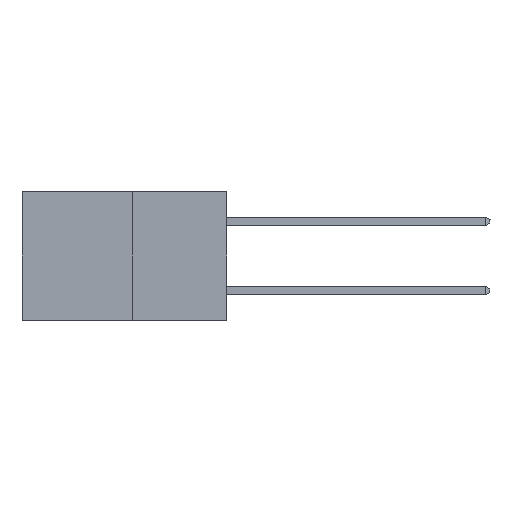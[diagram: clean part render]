
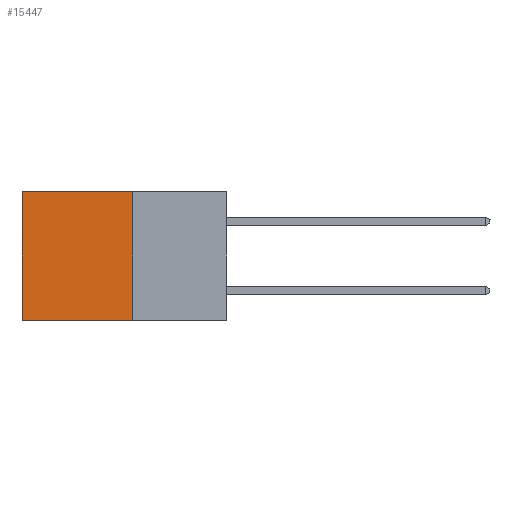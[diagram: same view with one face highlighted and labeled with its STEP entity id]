
A CAD part, left-side view. The second image highlights one B-rep face of the part: STEP entity #15447.
In plain terms, the highlighted planar face has unit normal (-1, 0, 0).
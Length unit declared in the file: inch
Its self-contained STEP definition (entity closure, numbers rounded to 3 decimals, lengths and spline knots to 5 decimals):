
#273 = FACE_OUTER_BOUND ( 'NONE', #14541, .T. ) ;
#446 = DIRECTION ( 'NONE',  ( 1., 0., 0. ) ) ;
#897 = EDGE_CURVE ( 'NONE', #8844, #6362, #9414, .T. ) ;
#1646 = CARTESIAN_POINT ( 'NONE',  ( 0.277, 0.59, -0.37 ) ) ;
#2128 = DIRECTION ( 'NONE',  ( 0., 1., 0. ) ) ;
#2238 = DIRECTION ( 'NONE',  ( 0., 0., -1. ) ) ;
#2495 = CARTESIAN_POINT ( 'NONE',  ( 0.277, 0.59, -0.37 ) ) ;
#2591 = CARTESIAN_POINT ( 'NONE',  ( 0.277, 0.27, -0.37 ) ) ;
#2794 = DIRECTION ( 'NONE',  ( 0., 1., 0. ) ) ;
#3604 = VECTOR ( 'NONE', #2794, 39.37008 ) ;
#4494 = LINE ( 'NONE', #2591, #3604 ) ;
#5032 = CARTESIAN_POINT ( 'NONE',  ( 0.277, 0.59, 0. ) ) ;
#5323 = LINE ( 'NONE', #15180, #15571 ) ;
#6038 = VECTOR ( 'NONE', #14435, 39.37008 ) ;
#6362 = VERTEX_POINT ( 'NONE', #15870 ) ;
#6744 = EDGE_CURVE ( 'NONE', #6362, #9347, #4494, .T. ) ;
#6822 = LINE ( 'NONE', #1646, #17434 ) ;
#7029 = VERTEX_POINT ( 'NONE', #5032 ) ;
#7453 = EDGE_CURVE ( 'NONE', #7029, #9347, #6822, .T. ) ;
#7504 = ORIENTED_EDGE ( 'NONE', *, *, #6744, .F. ) ;
#7928 = AXIS2_PLACEMENT_3D ( 'NONE', #13498, #446, #10574 ) ;
#8844 = VERTEX_POINT ( 'NONE', #16671 ) ;
#9106 = PLANE ( 'NONE',  #7928 ) ;
#9347 = VERTEX_POINT ( 'NONE', #2495 ) ;
#9414 = LINE ( 'NONE', #13975, #6038 ) ;
#10574 = DIRECTION ( 'NONE',  ( 0., 0., -1. ) ) ;
#12203 = ORIENTED_EDGE ( 'NONE', *, *, #12925, .T. ) ;
#12925 = EDGE_CURVE ( 'NONE', #8844, #7029, #5323, .T. ) ;
#13498 = CARTESIAN_POINT ( 'NONE',  ( 0.277, 0.27, -0.37 ) ) ;
#13975 = CARTESIAN_POINT ( 'NONE',  ( 0.277, 0.27, -0.37 ) ) ;
#14261 = ORIENTED_EDGE ( 'NONE', *, *, #7453, .T. ) ;
#14435 = DIRECTION ( 'NONE',  ( 0., 0., -1. ) ) ;
#14541 = EDGE_LOOP ( 'NONE', ( #14261, #7504, #14986, #12203 ) ) ;
#14986 = ORIENTED_EDGE ( 'NONE', *, *, #897, .F. ) ;
#15180 = CARTESIAN_POINT ( 'NONE',  ( 0.277, 0.27, 0. ) ) ;
#15447 = ADVANCED_FACE ( 'NONE', ( #273 ), #9106, .F. ) ;
#15571 = VECTOR ( 'NONE', #2128, 39.37008 ) ;
#15870 = CARTESIAN_POINT ( 'NONE',  ( 0.277, 0.27, -0.37 ) ) ;
#16671 = CARTESIAN_POINT ( 'NONE',  ( 0.277, 0.27, 0. ) ) ;
#17434 = VECTOR ( 'NONE', #2238, 39.37008 ) ;
